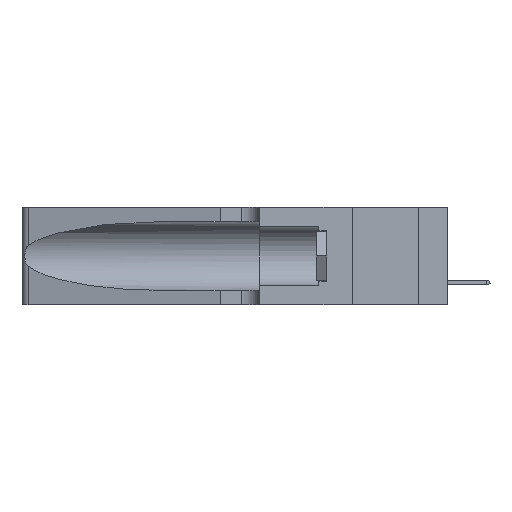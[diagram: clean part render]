
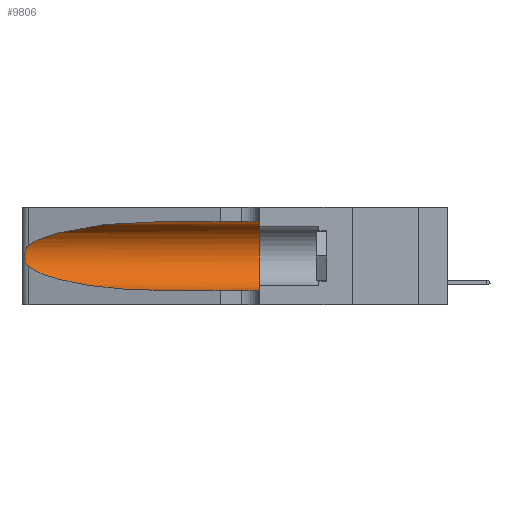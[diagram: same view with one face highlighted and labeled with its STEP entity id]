
A CAD part, left-side view. The second image highlights one B-rep face of the part: STEP entity #9806.
In plain terms, the highlighted cylindrical face has radius 3.308 mm (diameter 6.617 mm), a partial arc.
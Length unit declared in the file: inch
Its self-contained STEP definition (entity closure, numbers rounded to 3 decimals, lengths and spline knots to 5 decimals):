
#86 = CARTESIAN_POINT ( 'NONE',  ( 0.1305, 0.72297, 0.05475 ) ) ;
#95 = ORIENTED_EDGE ( 'NONE', *, *, #12738, .T. ) ;
#254 = EDGE_CURVE ( 'NONE', #17058, #1316, #9564, .T. ) ;
#410 = CARTESIAN_POINT ( 'NONE',  ( 0.1305, 1.61858, 0.185 ) ) ;
#876 = CARTESIAN_POINT ( 'NONE',  ( 0.25854, 1.2359, 0.20912 ) ) ;
#936 = CARTESIAN_POINT ( 'NONE',  ( 0.25856, 1.23593, 0.16098 ) ) ;
#996 = CARTESIAN_POINT ( 'NONE',  ( 0.26017, 1.23833, 0.17102 ) ) ;
#1316 = VERTEX_POINT ( 'NONE', #8416 ) ;
#1691 = ORIENTED_EDGE ( 'NONE', *, *, #7211, .T. ) ;
#1786 = CYLINDRICAL_SURFACE ( 'NONE', #17821, 0.13025 ) ;
#1971 = DIRECTION ( 'NONE',  ( 0., 1., 0. ) ) ;
#2420 = CARTESIAN_POINT ( 'NONE',  ( 0.25487, 1.22718, 0.14631 ) ) ;
#2489 = CARTESIAN_POINT ( 'NONE',  ( 0.25789, 1.23486, 0.15765 ) ) ;
#3187 = VERTEX_POINT ( 'NONE', #86 ) ;
#3366 = VERTEX_POINT ( 'NONE', #17804 ) ;
#3521 = ORIENTED_EDGE ( 'NONE', *, *, #254, .T. ) ;
#3973 = VERTEX_POINT ( 'NONE', #13771 ) ;
#4008 = CARTESIAN_POINT ( 'NONE',  ( 0.25787, 1.23484, 0.2124 ) ) ;
#4113 = CARTESIAN_POINT ( 'NONE',  ( 0.1305, 1.61858, 0.31525 ) ) ;
#4473 = CARTESIAN_POINT ( 'NONE',  ( 0.1305, 0.72297, 0.31525 ) ) ;
#4705 =( BOUNDED_CURVE ( )  B_SPLINE_CURVE ( 3, ( #16365, #7432, #13202, #5815 ),
 .UNSPECIFIED., .F., .T. ) 
 B_SPLINE_CURVE_WITH_KNOTS ( ( 4, 4 ),
 ( 3.44316, 4.71239 ),
 .UNSPECIFIED. ) 
 CURVE ( )  GEOMETRIC_REPRESENTATION_ITEM ( )  RATIONAL_B_SPLINE_CURVE ( ( 1., 0.87, 0.87, 1. ) ) 
 REPRESENTATION_ITEM ( '' )  );
#5012 = CARTESIAN_POINT ( 'NONE',  ( 0.25487, 1.22718, 0.22369 ) ) ;
#5238 = AXIS2_PLACEMENT_3D ( 'NONE', #15172, #1971, #9383 ) ;
#5244 = EDGE_CURVE ( 'NONE', #11339, #3973, #8895, .T. ) ;
#5315 =( BOUNDED_CURVE ( )  B_SPLINE_CURVE ( 3, ( #4473, #14643, #8877, #10338 ),
 .UNSPECIFIED., .F., .T. ) 
 B_SPLINE_CURVE_WITH_KNOTS ( ( 4, 4 ),
 ( 1.5708, 2.84003 ),
 .UNSPECIFIED. ) 
 CURVE ( )  GEOMETRIC_REPRESENTATION_ITEM ( )  RATIONAL_B_SPLINE_CURVE ( ( 1., 0.87, 0.87, 1. ) ) 
 REPRESENTATION_ITEM ( '' )  );
#5372 = CARTESIAN_POINT ( 'NONE',  ( 0.25555, 1.22994, 0.2215 ) ) ;
#5815 = CARTESIAN_POINT ( 'NONE',  ( 0.1305, 0.72297, 0.05475 ) ) ;
#6955 = ORIENTED_EDGE ( 'NONE', *, *, #17224, .F. ) ;
#7015 = CARTESIAN_POINT ( 'NONE',  ( 0.1305, 0.72297, 0.31525 ) ) ;
#7211 = EDGE_CURVE ( 'NONE', #11339, #17058, #5315, .T. ) ;
#7432 = CARTESIAN_POINT ( 'NONE',  ( 0.2373, 1.15595, 0.08982 ) ) ;
#7502 = VECTOR ( 'NONE', #17753, 39.37008 ) ;
#8416 = CARTESIAN_POINT ( 'NONE',  ( 0.25487, 1.22718, 0.14631 ) ) ;
#8877 = CARTESIAN_POINT ( 'NONE',  ( 0.2373, 1.15595, 0.28018 ) ) ;
#8895 = LINE ( 'NONE', #4113, #7502 ) ;
#9141 = DIRECTION ( 'NONE',  ( 0., -1., 0. ) ) ;
#9259 = CARTESIAN_POINT ( 'NONE',  ( 0.1305, 1.61858, 0.05475 ) ) ;
#9260 = VECTOR ( 'NONE', #9141, 39.37008 ) ;
#9383 = DIRECTION ( 'NONE',  ( 0., 0., 1. ) ) ;
#9564 = B_SPLINE_CURVE_WITH_KNOTS ( 'NONE', 3,
 ( #12654, #5372, #15675, #4008, #876, #18580, #17089, #9737, #996, #936, #2489, #11301, #11236, #2420 ),
 .UNSPECIFIED., .F., .F.,
 ( 4, 2, 2, 2, 2, 2, 4 ),
 ( 0., 0.00027, 0.00053, 0.00107, 0.0016, 0.00187, 0.00214 ),
 .UNSPECIFIED. ) ;
#9637 = FACE_OUTER_BOUND ( 'NONE', #10692, .T. ) ;
#9737 = CARTESIAN_POINT ( 'NONE',  ( 0.26075, 1.23896, 0.178 ) ) ;
#9806 = ADVANCED_FACE ( 'NONE', ( #9637 ), #1786, .F. ) ;
#10338 = CARTESIAN_POINT ( 'NONE',  ( 0.25487, 1.22718, 0.22369 ) ) ;
#10659 = DIRECTION ( 'NONE',  ( 0., -1., 0. ) ) ;
#10692 = EDGE_LOOP ( 'NONE', ( #1691, #3521, #12353, #95, #6955, #14189 ) ) ;
#11236 = CARTESIAN_POINT ( 'NONE',  ( 0.25555, 1.22993, 0.14849 ) ) ;
#11301 = CARTESIAN_POINT ( 'NONE',  ( 0.25639, 1.23186, 0.15144 ) ) ;
#11339 = VERTEX_POINT ( 'NONE', #7015 ) ;
#11612 = EDGE_CURVE ( 'NONE', #1316, #3187, #4705, .T. ) ;
#11785 = LINE ( 'NONE', #9259, #9260 ) ;
#12353 = ORIENTED_EDGE ( 'NONE', *, *, #11612, .T. ) ;
#12654 = CARTESIAN_POINT ( 'NONE',  ( 0.25487, 1.22718, 0.22369 ) ) ;
#12738 = EDGE_CURVE ( 'NONE', #3187, #3366, #11785, .T. ) ;
#13202 = CARTESIAN_POINT ( 'NONE',  ( 0.18966, 0.96281, 0.05475 ) ) ;
#13771 = CARTESIAN_POINT ( 'NONE',  ( 0.1305, 0.35, 0.31525 ) ) ;
#14189 = ORIENTED_EDGE ( 'NONE', *, *, #5244, .F. ) ;
#14380 = CIRCLE ( 'NONE', #5238, 0.13025 ) ;
#14643 = CARTESIAN_POINT ( 'NONE',  ( 0.18966, 0.96281, 0.31525 ) ) ;
#15161 = DIRECTION ( 'NONE',  ( 0., 0., -1. ) ) ;
#15172 = CARTESIAN_POINT ( 'NONE',  ( 0.1305, 0.35, 0.185 ) ) ;
#15675 = CARTESIAN_POINT ( 'NONE',  ( 0.25639, 1.23184, 0.21858 ) ) ;
#16365 = CARTESIAN_POINT ( 'NONE',  ( 0.25487, 1.22718, 0.14631 ) ) ;
#17058 = VERTEX_POINT ( 'NONE', #5012 ) ;
#17089 = CARTESIAN_POINT ( 'NONE',  ( 0.26075, 1.23896, 0.19203 ) ) ;
#17224 = EDGE_CURVE ( 'NONE', #3973, #3366, #14380, .T. ) ;
#17753 = DIRECTION ( 'NONE',  ( 0., -1., 0. ) ) ;
#17804 = CARTESIAN_POINT ( 'NONE',  ( 0.1305, 0.35, 0.05475 ) ) ;
#17821 = AXIS2_PLACEMENT_3D ( 'NONE', #410, #10659, #15161 ) ;
#18580 = CARTESIAN_POINT ( 'NONE',  ( 0.26018, 1.23835, 0.19895 ) ) ;
